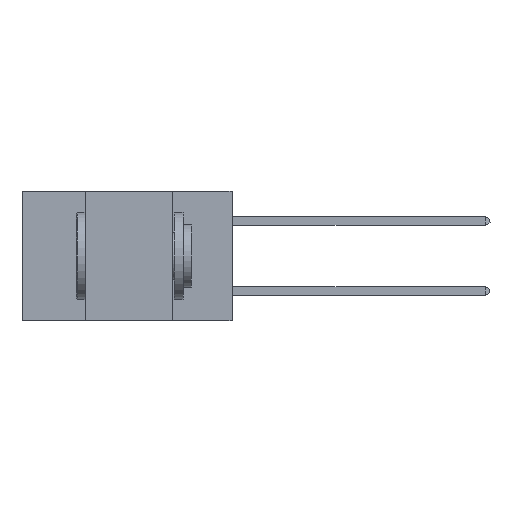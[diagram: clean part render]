
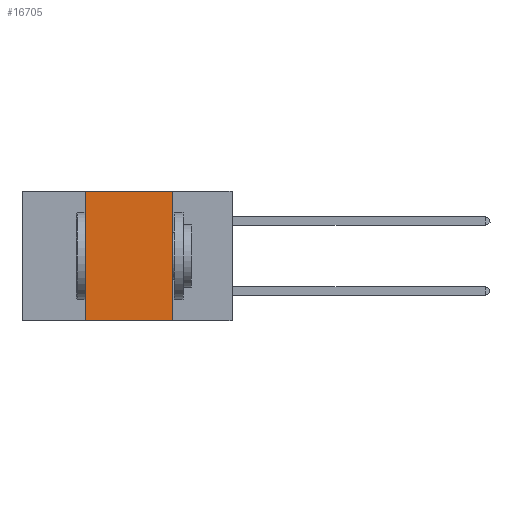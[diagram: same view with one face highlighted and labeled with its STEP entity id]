
A CAD part, left-side view. The second image highlights one B-rep face of the part: STEP entity #16705.
In plain terms, the highlighted planar face has unit normal (-1, 0, 0).
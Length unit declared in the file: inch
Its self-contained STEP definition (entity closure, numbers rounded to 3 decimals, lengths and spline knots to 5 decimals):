
#526 = CARTESIAN_POINT ( 'NONE',  ( 0., 0.42, 0. ) ) ;
#756 = CARTESIAN_POINT ( 'NONE',  ( 0., 0.6, 0. ) ) ;
#919 = DIRECTION ( 'NONE',  ( 0., -1., 0. ) ) ;
#1521 = LINE ( 'NONE', #18130, #16520 ) ;
#2180 = DIRECTION ( 'NONE',  ( 0., 0., -1. ) ) ;
#3352 = VERTEX_POINT ( 'NONE', #10542 ) ;
#3403 = CARTESIAN_POINT ( 'NONE',  ( 0., 0.42, -0.37 ) ) ;
#3711 = ORIENTED_EDGE ( 'NONE', *, *, #14470, .F. ) ;
#6100 = CARTESIAN_POINT ( 'NONE',  ( 0., 0.6, -0.37 ) ) ;
#6105 = VECTOR ( 'NONE', #9490, 39.37008 ) ;
#6823 = ORIENTED_EDGE ( 'NONE', *, *, #6888, .F. ) ;
#6888 = EDGE_CURVE ( 'NONE', #16166, #3352, #9920, .T. ) ;
#7321 = FACE_OUTER_BOUND ( 'NONE', #11274, .T. ) ;
#7651 = CARTESIAN_POINT ( 'NONE',  ( 0., 0.42, 0. ) ) ;
#8973 = EDGE_CURVE ( 'NONE', #14802, #13229, #16563, .T. ) ;
#9095 = VECTOR ( 'NONE', #13169, 39.37008 ) ;
#9358 = PLANE ( 'NONE',  #17546 ) ;
#9490 = DIRECTION ( 'NONE',  ( 0., 0., -1. ) ) ;
#9577 = ORIENTED_EDGE ( 'NONE', *, *, #8973, .F. ) ;
#9920 = LINE ( 'NONE', #13607, #6105 ) ;
#10370 = DIRECTION ( 'NONE',  ( 0., 0., 1. ) ) ;
#10542 = CARTESIAN_POINT ( 'NONE',  ( 0., 0.17, -0.37 ) ) ;
#10809 = DIRECTION ( 'NONE',  ( 1., 0., 0. ) ) ;
#11274 = EDGE_LOOP ( 'NONE', ( #6823, #3711, #9577, #15348 ) ) ;
#11565 = LINE ( 'NONE', #6100, #9095 ) ;
#11973 = EDGE_CURVE ( 'NONE', #14802, #3352, #11565, .T. ) ;
#13169 = DIRECTION ( 'NONE',  ( 0., -1., 0. ) ) ;
#13229 = VERTEX_POINT ( 'NONE', #526 ) ;
#13607 = CARTESIAN_POINT ( 'NONE',  ( 0., 0.17, 0. ) ) ;
#14470 = EDGE_CURVE ( 'NONE', #13229, #16166, #1521, .T. ) ;
#14802 = VERTEX_POINT ( 'NONE', #3403 ) ;
#15348 = ORIENTED_EDGE ( 'NONE', *, *, #11973, .T. ) ;
#15511 = CARTESIAN_POINT ( 'NONE',  ( 0., 0.17, 0. ) ) ;
#15685 = VECTOR ( 'NONE', #10370, 39.37008 ) ;
#16166 = VERTEX_POINT ( 'NONE', #15511 ) ;
#16520 = VECTOR ( 'NONE', #919, 39.37008 ) ;
#16563 = LINE ( 'NONE', #7651, #15685 ) ;
#16705 = ADVANCED_FACE ( 'NONE', ( #7321 ), #9358, .F. ) ;
#17546 = AXIS2_PLACEMENT_3D ( 'NONE', #756, #10809, #2180 ) ;
#18130 = CARTESIAN_POINT ( 'NONE',  ( 0., 0.6, 0. ) ) ;
